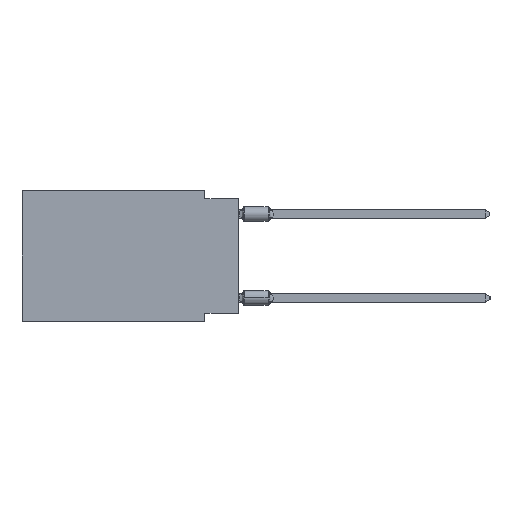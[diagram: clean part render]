
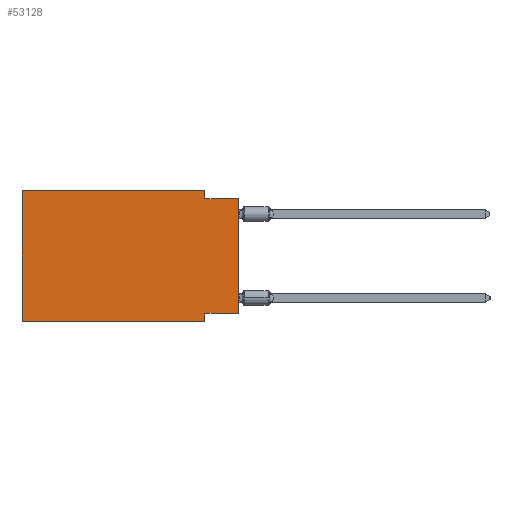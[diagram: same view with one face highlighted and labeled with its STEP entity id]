
A CAD part, left-side view. The second image highlights one B-rep face of the part: STEP entity #53128.
In plain terms, the highlighted planar face has unit normal (-1, 0, 0).
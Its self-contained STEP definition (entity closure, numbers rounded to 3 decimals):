
#2036 = EDGE_CURVE ( 'NONE', #34714, #29484, #32651, .T. ) ;
#2240 = EDGE_LOOP ( 'NONE', ( #35832, #29481, #20785, #39274, #6427, #48817, #37649, #7325 ) ) ;
#2771 = DIRECTION ( 'NONE',  ( 0., 1., 0. ) ) ;
#5073 = VERTEX_POINT ( 'NONE', #12953 ) ;
#5918 = DIRECTION ( 'NONE',  ( 0., 0., 1. ) ) ;
#6427 = ORIENTED_EDGE ( 'NONE', *, *, #28155, .F. ) ;
#7325 = ORIENTED_EDGE ( 'NONE', *, *, #45081, .F. ) ;
#7959 = VERTEX_POINT ( 'NONE', #14549 ) ;
#8183 = DIRECTION ( 'NONE',  ( 0., 0., -1. ) ) ;
#8705 = CARTESIAN_POINT ( 'NONE',  ( 0., 2.54, -9.271 ) ) ;
#9007 = CARTESIAN_POINT ( 'NONE',  ( 0., 0., 0. ) ) ;
#9287 = CARTESIAN_POINT ( 'NONE',  ( 0., 16.383, 0. ) ) ;
#10549 = DIRECTION ( 'NONE',  ( 0., 0., -1. ) ) ;
#11359 = CARTESIAN_POINT ( 'NONE',  ( 0., 0., -0.635 ) ) ;
#12953 = CARTESIAN_POINT ( 'NONE',  ( 0., 2.54, -0.635 ) ) ;
#14113 = VERTEX_POINT ( 'NONE', #11359 ) ;
#14549 = CARTESIAN_POINT ( 'NONE',  ( 0., 0., -9.271 ) ) ;
#15536 = FACE_OUTER_BOUND ( 'NONE', #2240, .T. ) ;
#15958 = LINE ( 'NONE', #23475, #45358 ) ;
#17801 = VERTEX_POINT ( 'NONE', #8705 ) ;
#19132 = VECTOR ( 'NONE', #54904, 1000. ) ;
#19521 = CARTESIAN_POINT ( 'NONE',  ( 0., 16.383, 0. ) ) ;
#20785 = ORIENTED_EDGE ( 'NONE', *, *, #44635, .F. ) ;
#21168 = CARTESIAN_POINT ( 'NONE',  ( 0., 16.383, 0. ) ) ;
#21853 = AXIS2_PLACEMENT_3D ( 'NONE', #32495, #48665, #10549 ) ;
#23475 = CARTESIAN_POINT ( 'NONE',  ( 0., 0., -0.635 ) ) ;
#25739 = VECTOR ( 'NONE', #2771, 1000. ) ;
#25961 = LINE ( 'NONE', #9287, #48947 ) ;
#27126 = VECTOR ( 'NONE', #53492, 1000. ) ;
#28150 = EDGE_CURVE ( 'NONE', #7959, #14113, #47391, .T. ) ;
#28155 = EDGE_CURVE ( 'NONE', #34714, #54965, #25961, .T. ) ;
#28707 = DIRECTION ( 'NONE',  ( 0., 0., -1. ) ) ;
#29481 = ORIENTED_EDGE ( 'NONE', *, *, #45813, .F. ) ;
#29484 = VERTEX_POINT ( 'NONE', #53766 ) ;
#30623 = CARTESIAN_POINT ( 'NONE',  ( 0., 16.383, -9.906 ) ) ;
#31682 = PLANE ( 'NONE',  #21853 ) ;
#32495 = CARTESIAN_POINT ( 'NONE',  ( 0., 16.383, 0. ) ) ;
#32539 = LINE ( 'NONE', #49521, #25739 ) ;
#32651 = LINE ( 'NONE', #45457, #19132 ) ;
#34313 = DIRECTION ( 'NONE',  ( 0., 0., 1. ) ) ;
#34714 = VERTEX_POINT ( 'NONE', #30623 ) ;
#35665 = EDGE_CURVE ( 'NONE', #54965, #46599, #49044, .T. ) ;
#35832 = ORIENTED_EDGE ( 'NONE', *, *, #28150, .T. ) ;
#37649 = ORIENTED_EDGE ( 'NONE', *, *, #54432, .F. ) ;
#39274 = ORIENTED_EDGE ( 'NONE', *, *, #35665, .F. ) ;
#40735 = DIRECTION ( 'NONE',  ( 0., -1., 0. ) ) ;
#44497 = VECTOR ( 'NONE', #5918, 1000. ) ;
#44635 = EDGE_CURVE ( 'NONE', #46599, #5073, #45419, .T. ) ;
#45081 = EDGE_CURVE ( 'NONE', #7959, #17801, #32539, .T. ) ;
#45358 = VECTOR ( 'NONE', #40735, 1000. ) ;
#45419 = LINE ( 'NONE', #53219, #52355 ) ;
#45457 = CARTESIAN_POINT ( 'NONE',  ( 0., 16.383, -9.906 ) ) ;
#45813 = EDGE_CURVE ( 'NONE', #5073, #14113, #15958, .T. ) ;
#46129 = CARTESIAN_POINT ( 'NONE',  ( 0., 2.54, 0. ) ) ;
#46599 = VERTEX_POINT ( 'NONE', #46129 ) ;
#47391 = LINE ( 'NONE', #9007, #44497 ) ;
#48594 = VECTOR ( 'NONE', #8183, 1000. ) ;
#48665 = DIRECTION ( 'NONE',  ( 1., 0., 0. ) ) ;
#48817 = ORIENTED_EDGE ( 'NONE', *, *, #2036, .T. ) ;
#48947 = VECTOR ( 'NONE', #34313, 1000. ) ;
#49044 = LINE ( 'NONE', #19521, #27126 ) ;
#49521 = CARTESIAN_POINT ( 'NONE',  ( 0., 0., -9.271 ) ) ;
#50466 = LINE ( 'NONE', #50746, #48594 ) ;
#50746 = CARTESIAN_POINT ( 'NONE',  ( 0., 2.54, -9.906 ) ) ;
#52355 = VECTOR ( 'NONE', #28707, 1000. ) ;
#53128 = ADVANCED_FACE ( 'NONE', ( #15536 ), #31682, .F. ) ;
#53219 = CARTESIAN_POINT ( 'NONE',  ( 0., 2.54, 0. ) ) ;
#53492 = DIRECTION ( 'NONE',  ( 0., -1., 0. ) ) ;
#53766 = CARTESIAN_POINT ( 'NONE',  ( 0., 2.54, -9.906 ) ) ;
#54432 = EDGE_CURVE ( 'NONE', #17801, #29484, #50466, .T. ) ;
#54904 = DIRECTION ( 'NONE',  ( 0., -1., 0. ) ) ;
#54965 = VERTEX_POINT ( 'NONE', #21168 ) ;
